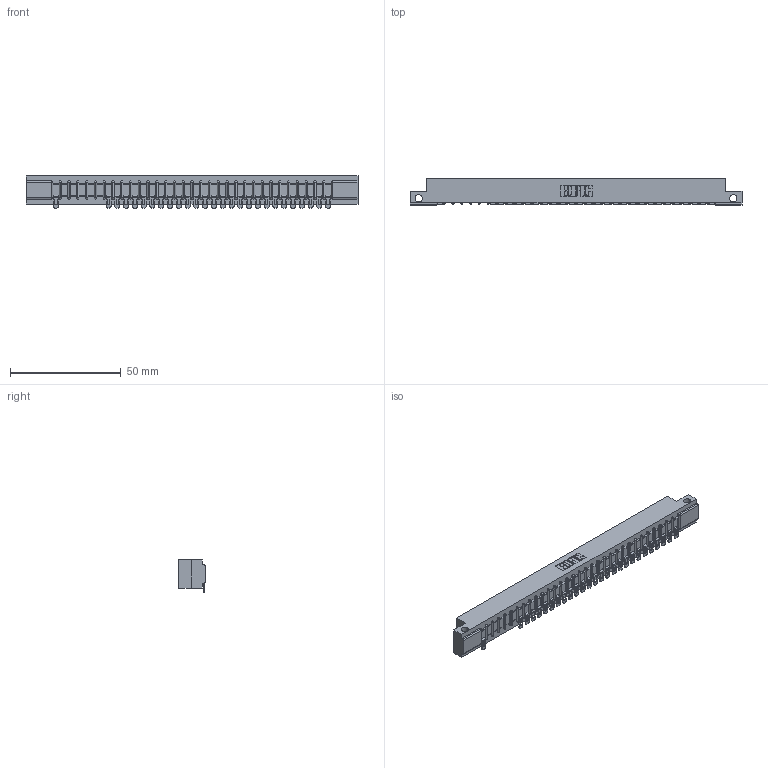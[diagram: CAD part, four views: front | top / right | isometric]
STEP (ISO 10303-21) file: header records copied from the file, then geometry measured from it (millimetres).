
FILE_DESCRIPTION (( 'STEP AP203' ), '1' );
FILE_NAME ('357-032-554-112.STEP', '2018-08-09T23:54:23', ( '' ), ( '' ), 'SwSTEP 2.0', 'SolidWorks 2016', '' );
FILE_SCHEMA (( 'CONFIG_CONTROL_DESIGN' ));
Length unit declared in the file: inch
Products named in the file (3): 307 Part_.128 Dia Side Mounting Holes; 307-290-002_554; 357-032-554-112
Assembly tree (28 placements, depth 2):
  357-032-554-112
    307 Part_.128 Dia Side Mounting Holes
    307-290-002_554  x27
Bounding box: 149.81 x 12.01 x 14.52 mm (x, y, z)
Volume: 15679.8 mm3; surface area: 18662.6 mm2
Topology: 28 solids, 28 shells, 2438 faces, 7474 edges, 4892 vertices
Faces by surface type: plane 1372, cylinder 1000, sphere 66
Entity records: 29473 total; most frequent: CARTESIAN_POINT 4993, ORIENTED_EDGE 4988, DIRECTION 4856, EDGE_CURVE 2494, VECTOR 1898, LINE 1898, VERTEX_POINT 1616, AXIS2_PLACEMENT_3D 1479
